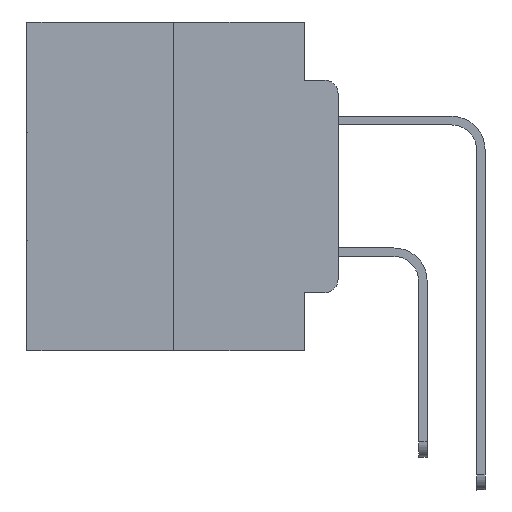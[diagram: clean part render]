
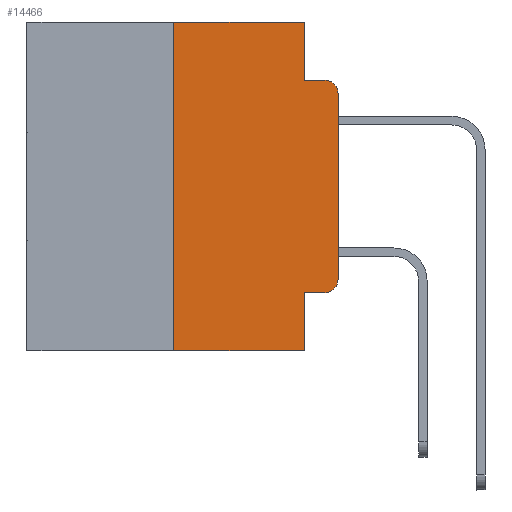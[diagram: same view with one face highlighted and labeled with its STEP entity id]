
A CAD part, left-side view. The second image highlights one B-rep face of the part: STEP entity #14466.
In plain terms, the highlighted planar face has unit normal (-1, 0, 0).
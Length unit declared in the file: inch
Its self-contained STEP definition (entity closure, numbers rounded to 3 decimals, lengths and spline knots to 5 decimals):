
#217 = ORIENTED_EDGE ( 'NONE', *, *, #13866, .F. ) ;
#750 = DIRECTION ( 'NONE',  ( 0., -1., 0. ) ) ;
#1057 = CARTESIAN_POINT ( 'NONE',  ( 0., 0.051, -0.0885 ) ) ;
#1132 = VERTEX_POINT ( 'NONE', #3004 ) ;
#2345 = DIRECTION ( 'NONE',  ( 0., 0., -1. ) ) ;
#2978 = CARTESIAN_POINT ( 'NONE',  ( 0., 0.25, 0. ) ) ;
#3004 = CARTESIAN_POINT ( 'NONE',  ( 0., 0.051, 0. ) ) ;
#3384 = VECTOR ( 'NONE', #19454, 39.37008 ) ;
#3788 = VERTEX_POINT ( 'NONE', #26245 ) ;
#3866 = LINE ( 'NONE', #5618, #22339 ) ;
#4041 = DIRECTION ( 'NONE',  ( 0., 0., 1. ) ) ;
#4125 = LINE ( 'NONE', #26226, #3384 ) ;
#4334 = VECTOR ( 'NONE', #22347, 39.37008 ) ;
#4614 = AXIS2_PLACEMENT_3D ( 'NONE', #7715, #26020, #12405 ) ;
#4842 = ORIENTED_EDGE ( 'NONE', *, *, #10703, .T. ) ;
#5618 = CARTESIAN_POINT ( 'NONE',  ( 0., 0.25, 0. ) ) ;
#7337 = EDGE_CURVE ( 'NONE', #18138, #14515, #23339, .T. ) ;
#7704 = ORIENTED_EDGE ( 'NONE', *, *, #25946, .T. ) ;
#7715 = CARTESIAN_POINT ( 'NONE',  ( 0., 0.473, 0. ) ) ;
#7860 = CARTESIAN_POINT ( 'NONE',  ( 0., 0.473, 0. ) ) ;
#8141 = CIRCLE ( 'NONE', #24990, 0.02 ) ;
#8521 = AXIS2_PLACEMENT_3D ( 'NONE', #11926, #27828, #14271 ) ;
#9373 = LINE ( 'NONE', #7860, #26881 ) ;
#10031 = VECTOR ( 'NONE', #4041, 39.37008 ) ;
#10703 = EDGE_CURVE ( 'NONE', #3788, #24474, #8141, .T. ) ;
#10830 = CARTESIAN_POINT ( 'NONE',  ( 0., 0.051, -0.4115 ) ) ;
#11108 = DIRECTION ( 'NONE',  ( 0., -1., 0. ) ) ;
#11182 = FACE_OUTER_BOUND ( 'NONE', #24143, .T. ) ;
#11592 = VECTOR ( 'NONE', #11108, 39.37008 ) ;
#11664 = VERTEX_POINT ( 'NONE', #2978 ) ;
#11926 = CARTESIAN_POINT ( 'NONE',  ( 0., 0.02, -0.1085 ) ) ;
#12222 = EDGE_CURVE ( 'NONE', #22538, #3788, #27340, .T. ) ;
#12356 = LINE ( 'NONE', #13949, #29748 ) ;
#12405 = DIRECTION ( 'NONE',  ( 0., 0., -1. ) ) ;
#13595 = DIRECTION ( 'NONE',  ( -1., 0., 0. ) ) ;
#13866 = EDGE_CURVE ( 'NONE', #11664, #1132, #9373, .T. ) ;
#13949 = CARTESIAN_POINT ( 'NONE',  ( 0., 0.051, 0. ) ) ;
#14271 = DIRECTION ( 'NONE',  ( 0., 0., -1. ) ) ;
#14466 = ADVANCED_FACE ( 'NONE', ( #11182 ), #23781, .F. ) ;
#14515 = VERTEX_POINT ( 'NONE', #17286 ) ;
#15070 = ORIENTED_EDGE ( 'NONE', *, *, #12222, .T. ) ;
#15344 = ORIENTED_EDGE ( 'NONE', *, *, #27460, .T. ) ;
#15351 = EDGE_CURVE ( 'NONE', #22538, #14515, #12356, .T. ) ;
#15950 = ORIENTED_EDGE ( 'NONE', *, *, #7337, .T. ) ;
#16191 = LINE ( 'NONE', #20269, #10031 ) ;
#16905 = EDGE_CURVE ( 'NONE', #18138, #11664, #3866, .T. ) ;
#17286 = CARTESIAN_POINT ( 'NONE',  ( 0., 0.051, -0.5 ) ) ;
#17400 = CARTESIAN_POINT ( 'NONE',  ( 0., 0.473, -0.5 ) ) ;
#18138 = VERTEX_POINT ( 'NONE', #25348 ) ;
#18418 = EDGE_CURVE ( 'NONE', #1132, #22820, #4125, .T. ) ;
#18687 = CARTESIAN_POINT ( 'NONE',  ( 0., 0.051, -0.4115 ) ) ;
#19454 = DIRECTION ( 'NONE',  ( 0., 0., -1. ) ) ;
#19658 = ORIENTED_EDGE ( 'NONE', *, *, #24472, .F. ) ;
#20269 = CARTESIAN_POINT ( 'NONE',  ( 0., 0., 0. ) ) ;
#20509 = ORIENTED_EDGE ( 'NONE', *, *, #15351, .F. ) ;
#21005 = VERTEX_POINT ( 'NONE', #24104 ) ;
#21742 = DIRECTION ( 'NONE',  ( 0., -1., 0. ) ) ;
#21766 = DIRECTION ( 'NONE',  ( 0., 0., 1. ) ) ;
#22339 = VECTOR ( 'NONE', #21766, 39.37008 ) ;
#22347 = DIRECTION ( 'NONE',  ( 0., -1., 0. ) ) ;
#22531 = CARTESIAN_POINT ( 'NONE',  ( 0., 0., -0.3915 ) ) ;
#22538 = VERTEX_POINT ( 'NONE', #18687 ) ;
#22820 = VERTEX_POINT ( 'NONE', #1057 ) ;
#23339 = LINE ( 'NONE', #17400, #28635 ) ;
#23781 = PLANE ( 'NONE',  #4614 ) ;
#24104 = CARTESIAN_POINT ( 'NONE',  ( 0., 0.02, -0.0885 ) ) ;
#24143 = EDGE_LOOP ( 'NONE', ( #15344, #7704, #19658, #25314, #217, #27910, #15950, #20509, #15070, #4842 ) ) ;
#24472 = EDGE_CURVE ( 'NONE', #22820, #21005, #29058, .T. ) ;
#24474 = VERTEX_POINT ( 'NONE', #22531 ) ;
#24782 = CARTESIAN_POINT ( 'NONE',  ( 0., 0.051, -0.0885 ) ) ;
#24990 = AXIS2_PLACEMENT_3D ( 'NONE', #27177, #13595, #29442 ) ;
#25314 = ORIENTED_EDGE ( 'NONE', *, *, #18418, .F. ) ;
#25348 = CARTESIAN_POINT ( 'NONE',  ( 0., 0.25, -0.5 ) ) ;
#25946 = EDGE_CURVE ( 'NONE', #26194, #21005, #26424, .T. ) ;
#26020 = DIRECTION ( 'NONE',  ( 1., 0., 0. ) ) ;
#26194 = VERTEX_POINT ( 'NONE', #26746 ) ;
#26226 = CARTESIAN_POINT ( 'NONE',  ( 0., 0.051, 0. ) ) ;
#26245 = CARTESIAN_POINT ( 'NONE',  ( 0., 0.02, -0.4115 ) ) ;
#26424 = CIRCLE ( 'NONE', #8521, 0.02 ) ;
#26746 = CARTESIAN_POINT ( 'NONE',  ( 0., 0., -0.1085 ) ) ;
#26881 = VECTOR ( 'NONE', #750, 39.37008 ) ;
#27177 = CARTESIAN_POINT ( 'NONE',  ( 0., 0.02, -0.3915 ) ) ;
#27340 = LINE ( 'NONE', #10830, #4334 ) ;
#27460 = EDGE_CURVE ( 'NONE', #24474, #26194, #16191, .T. ) ;
#27828 = DIRECTION ( 'NONE',  ( -1., 0., 0. ) ) ;
#27910 = ORIENTED_EDGE ( 'NONE', *, *, #16905, .F. ) ;
#28635 = VECTOR ( 'NONE', #21742, 39.37008 ) ;
#29058 = LINE ( 'NONE', #24782, #11592 ) ;
#29442 = DIRECTION ( 'NONE',  ( 0., 0., -1. ) ) ;
#29748 = VECTOR ( 'NONE', #2345, 39.37008 ) ;
